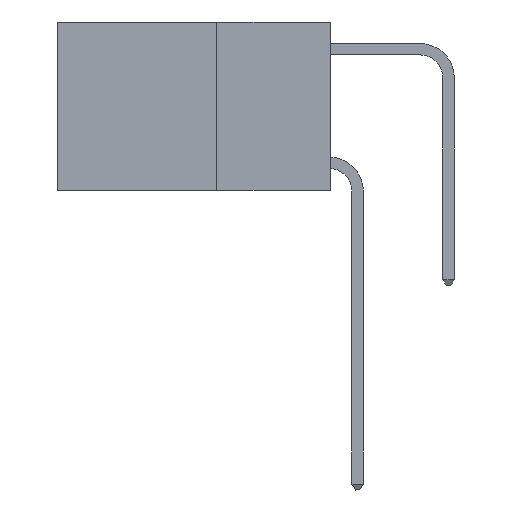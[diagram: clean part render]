
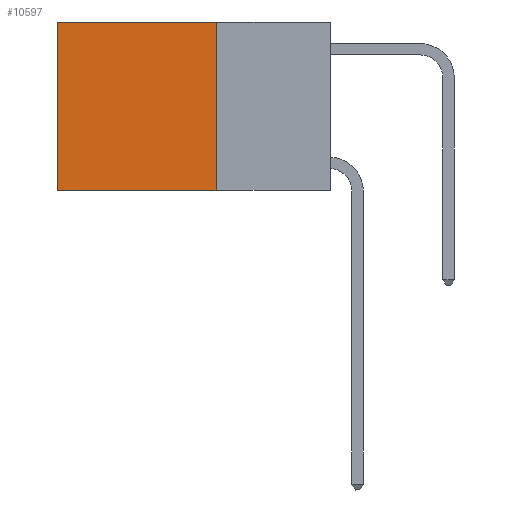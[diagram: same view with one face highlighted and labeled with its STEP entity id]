
A CAD part, left-side view. The second image highlights one B-rep face of the part: STEP entity #10597.
In plain terms, the highlighted planar face has unit normal (-1, 0, 0).
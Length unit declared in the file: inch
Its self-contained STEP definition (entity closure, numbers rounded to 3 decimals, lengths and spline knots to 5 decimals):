
#35 = VERTEX_POINT ( 'NONE', #5080 ) ;
#44 = VERTEX_POINT ( 'NONE', #4916 ) ;
#77 = EDGE_CURVE ( 'NONE', #35, #3184, #6204, .T. ) ;
#133 = ORIENTED_EDGE ( 'NONE', *, *, #2622, .T. ) ;
#1102 = PLANE ( 'NONE',  #10699 ) ;
#1711 = VECTOR ( 'NONE', #6201, 39.37008 ) ;
#1905 = FACE_OUTER_BOUND ( 'NONE', #4708, .T. ) ;
#2391 = CARTESIAN_POINT ( 'NONE',  ( 0.2625, 0.6, -0.37 ) ) ;
#2612 = CARTESIAN_POINT ( 'NONE',  ( 0.2625, 0.25, 0. ) ) ;
#2622 = EDGE_CURVE ( 'NONE', #44, #35, #11340, .T. ) ;
#2957 = VERTEX_POINT ( 'NONE', #8658 ) ;
#3184 = VERTEX_POINT ( 'NONE', #2391 ) ;
#3280 = EDGE_CURVE ( 'NONE', #44, #2957, #7385, .T. ) ;
#3743 = ORIENTED_EDGE ( 'NONE', *, *, #3280, .F. ) ;
#4083 = DIRECTION ( 'NONE',  ( 1., 0., 0. ) ) ;
#4579 = DIRECTION ( 'NONE',  ( 0., 1., 0. ) ) ;
#4683 = DIRECTION ( 'NONE',  ( 0., 0., -1. ) ) ;
#4689 = CARTESIAN_POINT ( 'NONE',  ( 0.2625, 0.6, 0. ) ) ;
#4708 = EDGE_LOOP ( 'NONE', ( #7446, #11493, #3743, #133 ) ) ;
#4745 = EDGE_CURVE ( 'NONE', #2957, #3184, #6781, .T. ) ;
#4916 = CARTESIAN_POINT ( 'NONE',  ( 0.2625, 0.25, 0. ) ) ;
#5080 = CARTESIAN_POINT ( 'NONE',  ( 0.2625, 0.6, 0. ) ) ;
#5263 = VECTOR ( 'NONE', #9126, 39.37008 ) ;
#6201 = DIRECTION ( 'NONE',  ( 0., 1., 0. ) ) ;
#6204 = LINE ( 'NONE', #4689, #8895 ) ;
#6781 = LINE ( 'NONE', #11607, #1711 ) ;
#7302 = CARTESIAN_POINT ( 'NONE',  ( 0.2625, 0.25, 0. ) ) ;
#7385 = LINE ( 'NONE', #2612, #5263 ) ;
#7446 = ORIENTED_EDGE ( 'NONE', *, *, #77, .T. ) ;
#8658 = CARTESIAN_POINT ( 'NONE',  ( 0.2625, 0.25, -0.37 ) ) ;
#8895 = VECTOR ( 'NONE', #4683, 39.37008 ) ;
#8959 = VECTOR ( 'NONE', #4579, 39.37008 ) ;
#9126 = DIRECTION ( 'NONE',  ( 0., 0., -1. ) ) ;
#9600 = CARTESIAN_POINT ( 'NONE',  ( 0.2625, 0.25, 0. ) ) ;
#10516 = DIRECTION ( 'NONE',  ( 0., 0., -1. ) ) ;
#10597 = ADVANCED_FACE ( 'NONE', ( #1905 ), #1102, .F. ) ;
#10699 = AXIS2_PLACEMENT_3D ( 'NONE', #9600, #4083, #10516 ) ;
#11340 = LINE ( 'NONE', #7302, #8959 ) ;
#11493 = ORIENTED_EDGE ( 'NONE', *, *, #4745, .F. ) ;
#11607 = CARTESIAN_POINT ( 'NONE',  ( 0.2625, 0.25, -0.37 ) ) ;
